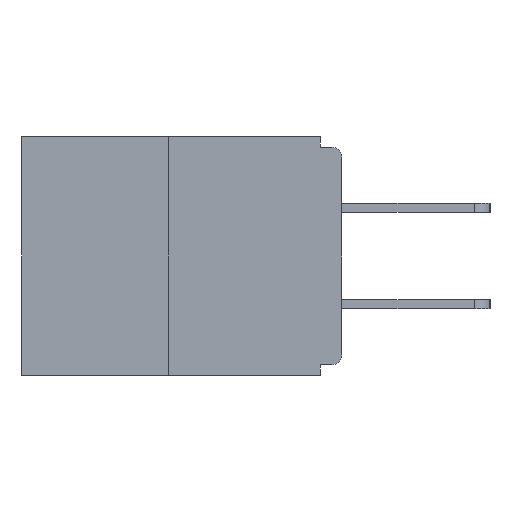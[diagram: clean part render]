
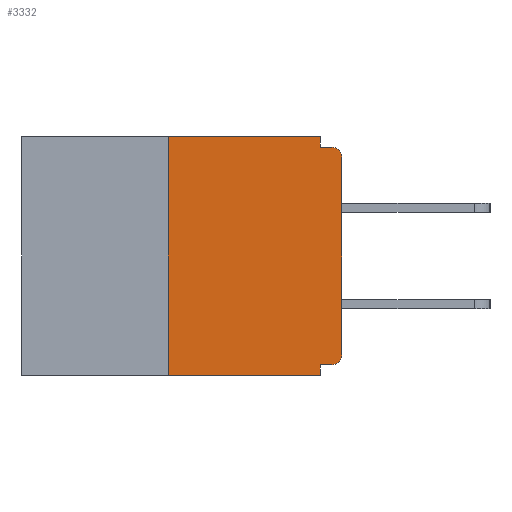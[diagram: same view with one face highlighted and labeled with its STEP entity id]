
A CAD part, left-side view. The second image highlights one B-rep face of the part: STEP entity #3332.
In plain terms, the highlighted planar face has unit normal (-1, 0, 0).
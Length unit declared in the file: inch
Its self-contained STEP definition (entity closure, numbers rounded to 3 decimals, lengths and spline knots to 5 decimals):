
#138 = LINE ( 'NONE', #6995, #4596 ) ;
#200 = VECTOR ( 'NONE', #6231, 39.37008 ) ;
#287 = CARTESIAN_POINT ( 'NONE',  ( 0., 0.031, -0.328 ) ) ;
#337 = CARTESIAN_POINT ( 'NONE',  ( 0., 0.031, 0. ) ) ;
#354 = VERTEX_POINT ( 'NONE', #3523 ) ;
#372 = CARTESIAN_POINT ( 'NONE',  ( 0., 0.46, 0. ) ) ;
#415 = VECTOR ( 'NONE', #7487, 39.37008 ) ;
#500 = EDGE_CURVE ( 'NONE', #9328, #7740, #1184, .T. ) ;
#542 = DIRECTION ( 'NONE',  ( 0., 0., -1. ) ) ;
#698 = VERTEX_POINT ( 'NONE', #10560 ) ;
#762 = LINE ( 'NONE', #11022, #4767 ) ;
#1054 = DIRECTION ( 'NONE',  ( 0., 0., 1. ) ) ;
#1113 = DIRECTION ( 'NONE',  ( 0., 0., 1. ) ) ;
#1115 = CARTESIAN_POINT ( 'NONE',  ( 0., 0.031, -0.015 ) ) ;
#1184 = LINE ( 'NONE', #372, #200 ) ;
#1606 = CIRCLE ( 'NONE', #6973, 0.015 ) ;
#1893 = EDGE_CURVE ( 'NONE', #7776, #698, #5898, .T. ) ;
#2235 = VECTOR ( 'NONE', #1113, 39.37008 ) ;
#2348 = CARTESIAN_POINT ( 'NONE',  ( 0., 0., -0.015 ) ) ;
#2631 = EDGE_CURVE ( 'NONE', #10645, #8269, #4602, .T. ) ;
#2686 = CIRCLE ( 'NONE', #10130, 0.015 ) ;
#2758 = EDGE_CURVE ( 'NONE', #7740, #5736, #762, .T. ) ;
#2845 = DIRECTION ( 'NONE',  ( -1., 0., 0. ) ) ;
#3003 = EDGE_CURVE ( 'NONE', #3411, #9328, #138, .T. ) ;
#3092 = CARTESIAN_POINT ( 'NONE',  ( 0., 0., -0.03 ) ) ;
#3248 = CARTESIAN_POINT ( 'NONE',  ( 0., 0.015, -0.03 ) ) ;
#3332 = ADVANCED_FACE ( 'NONE', ( #10813 ), #7360, .F. ) ;
#3411 = VERTEX_POINT ( 'NONE', #10126 ) ;
#3523 = CARTESIAN_POINT ( 'NONE',  ( 0., 0.015, -0.015 ) ) ;
#3570 = DIRECTION ( 'NONE',  ( 0., -1., 0. ) ) ;
#3712 = ORIENTED_EDGE ( 'NONE', *, *, #1893, .F. ) ;
#3984 = VERTEX_POINT ( 'NONE', #8009 ) ;
#4057 = ORIENTED_EDGE ( 'NONE', *, *, #9867, .T. ) ;
#4154 = DIRECTION ( 'NONE',  ( 0., 0., -1. ) ) ;
#4205 = DIRECTION ( 'NONE',  ( -1., 0., 0. ) ) ;
#4596 = VECTOR ( 'NONE', #1054, 39.37008 ) ;
#4602 = LINE ( 'NONE', #8878, #2235 ) ;
#4767 = VECTOR ( 'NONE', #542, 39.37008 ) ;
#5090 = EDGE_CURVE ( 'NONE', #8269, #354, #1606, .T. ) ;
#5103 = AXIS2_PLACEMENT_3D ( 'NONE', #5458, #9131, #7415 ) ;
#5323 = ORIENTED_EDGE ( 'NONE', *, *, #5090, .T. ) ;
#5458 = CARTESIAN_POINT ( 'NONE',  ( 0., 0.46, 0. ) ) ;
#5736 = VERTEX_POINT ( 'NONE', #1115 ) ;
#5898 = LINE ( 'NONE', #8331, #415 ) ;
#5927 = LINE ( 'NONE', #9391, #10499 ) ;
#6119 = ORIENTED_EDGE ( 'NONE', *, *, #2758, .F. ) ;
#6231 = DIRECTION ( 'NONE',  ( 0., -1., 0. ) ) ;
#6295 = ORIENTED_EDGE ( 'NONE', *, *, #3003, .F. ) ;
#6329 = DIRECTION ( 'NONE',  ( 0., 0., -1. ) ) ;
#6634 = ORIENTED_EDGE ( 'NONE', *, *, #8998, .F. ) ;
#6645 = EDGE_LOOP ( 'NONE', ( #8629, #6295, #9837, #3712, #6634, #4057, #8317, #5323, #8622, #6119 ) ) ;
#6747 = DIRECTION ( 'NONE',  ( 0., -1., 0. ) ) ;
#6973 = AXIS2_PLACEMENT_3D ( 'NONE', #3248, #4205, #4154 ) ;
#6995 = CARTESIAN_POINT ( 'NONE',  ( 0., 0.25, 0. ) ) ;
#7360 = PLANE ( 'NONE',  #5103 ) ;
#7373 = LINE ( 'NONE', #10829, #8871 ) ;
#7415 = DIRECTION ( 'NONE',  ( 0., 0., -1. ) ) ;
#7487 = DIRECTION ( 'NONE',  ( 0., 0., -1. ) ) ;
#7589 = LINE ( 'NONE', #2348, #9616 ) ;
#7740 = VERTEX_POINT ( 'NONE', #337 ) ;
#7776 = VERTEX_POINT ( 'NONE', #287 ) ;
#8009 = CARTESIAN_POINT ( 'NONE',  ( 0., 0.015, -0.328 ) ) ;
#8204 = CARTESIAN_POINT ( 'NONE',  ( 0., 0.25, 0. ) ) ;
#8269 = VERTEX_POINT ( 'NONE', #3092 ) ;
#8317 = ORIENTED_EDGE ( 'NONE', *, *, #2631, .T. ) ;
#8323 = EDGE_CURVE ( 'NONE', #5736, #354, #7589, .T. ) ;
#8331 = CARTESIAN_POINT ( 'NONE',  ( 0., 0.031, -0.343 ) ) ;
#8461 = CARTESIAN_POINT ( 'NONE',  ( 0., 0., -0.313 ) ) ;
#8622 = ORIENTED_EDGE ( 'NONE', *, *, #8323, .F. ) ;
#8629 = ORIENTED_EDGE ( 'NONE', *, *, #500, .F. ) ;
#8871 = VECTOR ( 'NONE', #10886, 39.37008 ) ;
#8878 = CARTESIAN_POINT ( 'NONE',  ( 0., 0., 0. ) ) ;
#8998 = EDGE_CURVE ( 'NONE', #3984, #7776, #7373, .T. ) ;
#9131 = DIRECTION ( 'NONE',  ( 1., 0., 0. ) ) ;
#9328 = VERTEX_POINT ( 'NONE', #8204 ) ;
#9391 = CARTESIAN_POINT ( 'NONE',  ( 0., 0.46, -0.343 ) ) ;
#9616 = VECTOR ( 'NONE', #6747, 39.37008 ) ;
#9837 = ORIENTED_EDGE ( 'NONE', *, *, #10085, .T. ) ;
#9867 = EDGE_CURVE ( 'NONE', #3984, #10645, #2686, .T. ) ;
#10085 = EDGE_CURVE ( 'NONE', #3411, #698, #5927, .T. ) ;
#10126 = CARTESIAN_POINT ( 'NONE',  ( 0., 0.25, -0.343 ) ) ;
#10130 = AXIS2_PLACEMENT_3D ( 'NONE', #10569, #2845, #6329 ) ;
#10499 = VECTOR ( 'NONE', #3570, 39.37008 ) ;
#10560 = CARTESIAN_POINT ( 'NONE',  ( 0., 0.031, -0.343 ) ) ;
#10569 = CARTESIAN_POINT ( 'NONE',  ( 0., 0.015, -0.313 ) ) ;
#10645 = VERTEX_POINT ( 'NONE', #8461 ) ;
#10813 = FACE_OUTER_BOUND ( 'NONE', #6645, .T. ) ;
#10829 = CARTESIAN_POINT ( 'NONE',  ( 0., 0., -0.328 ) ) ;
#10886 = DIRECTION ( 'NONE',  ( 0., 1., 0. ) ) ;
#11022 = CARTESIAN_POINT ( 'NONE',  ( 0., 0.031, 0. ) ) ;
